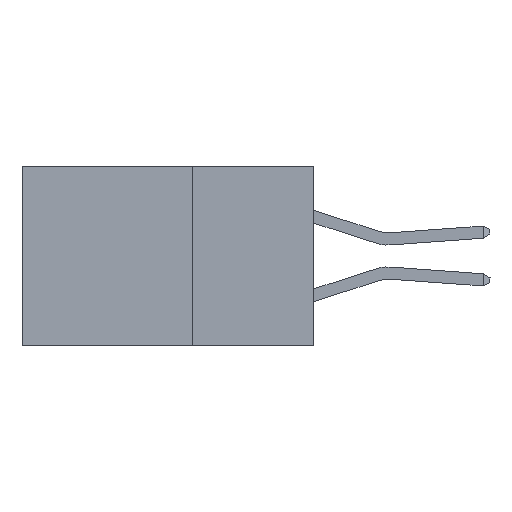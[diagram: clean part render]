
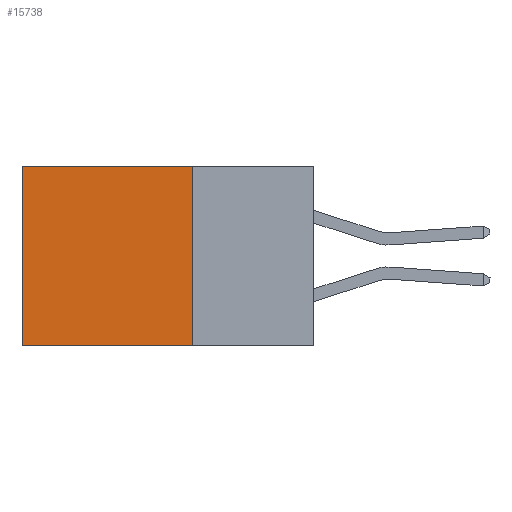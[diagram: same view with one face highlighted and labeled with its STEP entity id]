
A CAD part, left-side view. The second image highlights one B-rep face of the part: STEP entity #15738.
In plain terms, the highlighted planar face has unit normal (-1, 0, 0).
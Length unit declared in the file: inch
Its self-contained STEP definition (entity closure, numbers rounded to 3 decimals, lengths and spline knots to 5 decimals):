
#572 = ORIENTED_EDGE ( 'NONE', *, *, #2250, .F. ) ;
#902 = ORIENTED_EDGE ( 'NONE', *, *, #3489, .T. ) ;
#1591 = CARTESIAN_POINT ( 'NONE',  ( 0.2875, 0.25, -0.37 ) ) ;
#2250 = EDGE_CURVE ( 'NONE', #6558, #15804, #3929, .T. ) ;
#2497 = VERTEX_POINT ( 'NONE', #14886 ) ;
#2550 = DIRECTION ( 'NONE',  ( 1., 0., 0. ) ) ;
#3086 = VECTOR ( 'NONE', #3350, 39.37008 ) ;
#3350 = DIRECTION ( 'NONE',  ( 0., 0., -1. ) ) ;
#3474 = VECTOR ( 'NONE', #6046, 39.37008 ) ;
#3489 = EDGE_CURVE ( 'NONE', #6558, #2497, #13214, .T. ) ;
#3808 = DIRECTION ( 'NONE',  ( 0., 1., 0. ) ) ;
#3916 = CARTESIAN_POINT ( 'NONE',  ( 0.2875, 0.25, 0. ) ) ;
#3929 = LINE ( 'NONE', #3941, #3086 ) ;
#3941 = CARTESIAN_POINT ( 'NONE',  ( 0.2875, 0.25, 0. ) ) ;
#4671 = EDGE_CURVE ( 'NONE', #2497, #7904, #7182, .T. ) ;
#5595 = LINE ( 'NONE', #1591, #11971 ) ;
#5985 = CARTESIAN_POINT ( 'NONE',  ( 0.2875, 0.6, 0. ) ) ;
#6046 = DIRECTION ( 'NONE',  ( 0., 0., -1. ) ) ;
#6558 = VERTEX_POINT ( 'NONE', #12020 ) ;
#6743 = PLANE ( 'NONE',  #7657 ) ;
#6826 = EDGE_CURVE ( 'NONE', #15804, #7904, #5595, .T. ) ;
#6917 = CARTESIAN_POINT ( 'NONE',  ( 0.2875, 0.25, -0.37 ) ) ;
#7182 = LINE ( 'NONE', #5985, #3474 ) ;
#7289 = DIRECTION ( 'NONE',  ( 0., 1., 0. ) ) ;
#7657 = AXIS2_PLACEMENT_3D ( 'NONE', #10854, #2550, #12166 ) ;
#7904 = VERTEX_POINT ( 'NONE', #14511 ) ;
#8962 = ORIENTED_EDGE ( 'NONE', *, *, #4671, .T. ) ;
#9334 = ORIENTED_EDGE ( 'NONE', *, *, #6826, .F. ) ;
#10204 = VECTOR ( 'NONE', #3808, 39.37008 ) ;
#10854 = CARTESIAN_POINT ( 'NONE',  ( 0.2875, 0.25, 0. ) ) ;
#11971 = VECTOR ( 'NONE', #7289, 39.37008 ) ;
#12020 = CARTESIAN_POINT ( 'NONE',  ( 0.2875, 0.25, 0. ) ) ;
#12166 = DIRECTION ( 'NONE',  ( 0., 0., -1. ) ) ;
#12551 = FACE_OUTER_BOUND ( 'NONE', #13523, .T. ) ;
#13214 = LINE ( 'NONE', #3916, #10204 ) ;
#13523 = EDGE_LOOP ( 'NONE', ( #8962, #9334, #572, #902 ) ) ;
#14511 = CARTESIAN_POINT ( 'NONE',  ( 0.2875, 0.6, -0.37 ) ) ;
#14886 = CARTESIAN_POINT ( 'NONE',  ( 0.2875, 0.6, 0. ) ) ;
#15738 = ADVANCED_FACE ( 'NONE', ( #12551 ), #6743, .F. ) ;
#15804 = VERTEX_POINT ( 'NONE', #6917 ) ;
